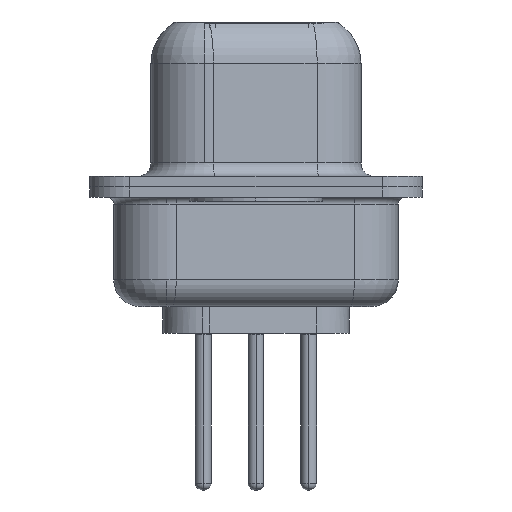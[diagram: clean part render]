
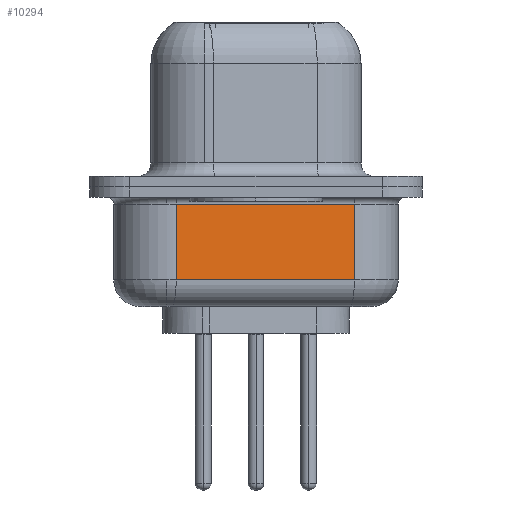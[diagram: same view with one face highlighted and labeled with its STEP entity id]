
A CAD part, left-side view. The second image highlights one B-rep face of the part: STEP entity #10294.
In plain terms, the highlighted planar face has unit normal (-0.985, -0.174, 0).
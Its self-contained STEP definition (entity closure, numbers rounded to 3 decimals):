
#266 = DIRECTION ( 'NONE',  ( 0., 0., 1. ) ) ;
#601 = EDGE_CURVE ( 'NONE', #5438, #24844, #20117, .T. ) ;
#693 = DIRECTION ( 'NONE',  ( -0.174, 0.985, 0. ) ) ;
#1437 = CARTESIAN_POINT ( 'NONE',  ( 4.037, -3.697, -0.65 ) ) ;
#2723 = LINE ( 'NONE', #26907, #3358 ) ;
#3054 = LINE ( 'NONE', #5078, #6447 ) ;
#3087 = EDGE_CURVE ( 'NONE', #24844, #14261, #17865, .T. ) ;
#3358 = VECTOR ( 'NONE', #693, 1000. ) ;
#4711 = AXIS2_PLACEMENT_3D ( 'NONE', #13646, #9114, #15959 ) ;
#5078 = CARTESIAN_POINT ( 'NONE',  ( 2.855, 3.003, -4.5 ) ) ;
#5438 = VERTEX_POINT ( 'NONE', #20705 ) ;
#6447 = VECTOR ( 'NONE', #9166, 1000. ) ;
#7063 = PLANE ( 'NONE',  #4711 ) ;
#9114 = DIRECTION ( 'NONE',  ( 0.985, 0.174, 0. ) ) ;
#9166 = DIRECTION ( 'NONE',  ( 0., 0., 1. ) ) ;
#9885 = VECTOR ( 'NONE', #266, 1000. ) ;
#9927 = ORIENTED_EDGE ( 'NONE', *, *, #23642, .F. ) ;
#10294 = ADVANCED_FACE ( 'NONE', ( #20186 ), #7063, .F. ) ;
#10688 = EDGE_CURVE ( 'NONE', #14261, #20653, #2723, .T. ) ;
#10940 = CARTESIAN_POINT ( 'NONE',  ( 2.855, 3.003, -0.65 ) ) ;
#11315 = CARTESIAN_POINT ( 'NONE',  ( 4.037, -3.697, -4.5 ) ) ;
#12029 = ORIENTED_EDGE ( 'NONE', *, *, #3087, .T. ) ;
#12491 = EDGE_LOOP ( 'NONE', ( #9927, #24878, #12029, #22224 ) ) ;
#13294 = DIRECTION ( 'NONE',  ( 0.174, -0.985, 0. ) ) ;
#13646 = CARTESIAN_POINT ( 'NONE',  ( 2.855, 3.003, -4.5 ) ) ;
#14261 = VERTEX_POINT ( 'NONE', #1437 ) ;
#15748 = CARTESIAN_POINT ( 'NONE',  ( 2.855, 3.003, -3.5 ) ) ;
#15959 = DIRECTION ( 'NONE',  ( -0.174, 0.985, 0. ) ) ;
#17865 = LINE ( 'NONE', #11315, #9885 ) ;
#20117 = LINE ( 'NONE', #15748, #28079 ) ;
#20186 = FACE_OUTER_BOUND ( 'NONE', #12491, .T. ) ;
#20653 = VERTEX_POINT ( 'NONE', #10940 ) ;
#20705 = CARTESIAN_POINT ( 'NONE',  ( 2.855, 3.003, -3.5 ) ) ;
#22224 = ORIENTED_EDGE ( 'NONE', *, *, #10688, .T. ) ;
#23642 = EDGE_CURVE ( 'NONE', #5438, #20653, #3054, .T. ) ;
#24844 = VERTEX_POINT ( 'NONE', #28135 ) ;
#24878 = ORIENTED_EDGE ( 'NONE', *, *, #601, .T. ) ;
#26907 = CARTESIAN_POINT ( 'NONE',  ( 2.855, 3.003, -0.65 ) ) ;
#28079 = VECTOR ( 'NONE', #13294, 1000. ) ;
#28135 = CARTESIAN_POINT ( 'NONE',  ( 4.037, -3.697, -3.5 ) ) ;
